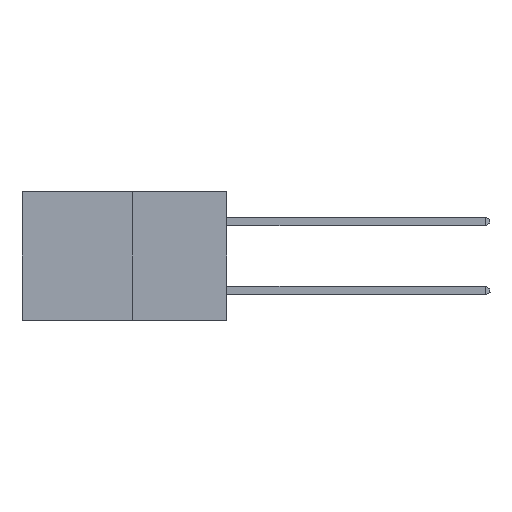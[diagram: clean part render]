
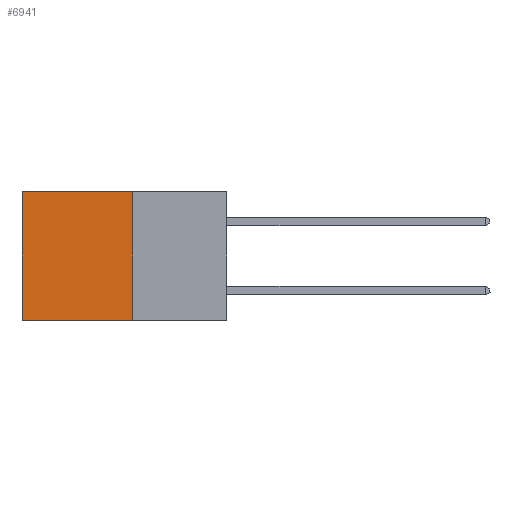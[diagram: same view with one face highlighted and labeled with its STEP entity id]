
A CAD part, left-side view. The second image highlights one B-rep face of the part: STEP entity #6941.
In plain terms, the highlighted planar face has unit normal (-1, 0, 0).
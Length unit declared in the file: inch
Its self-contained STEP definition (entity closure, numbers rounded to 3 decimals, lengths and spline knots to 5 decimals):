
#13 = CARTESIAN_POINT ( 'NONE',  ( 0.277, 0.27, 0. ) ) ;
#68 = LINE ( 'NONE', #5276, #3127 ) ;
#128 = ORIENTED_EDGE ( 'NONE', *, *, #6680, .T. ) ;
#270 = PLANE ( 'NONE',  #3419 ) ;
#528 = EDGE_CURVE ( 'NONE', #2380, #3860, #68, .T. ) ;
#669 = DIRECTION ( 'NONE',  ( 0., 1., 0. ) ) ;
#721 = DIRECTION ( 'NONE',  ( 0., 0., -1. ) ) ;
#1152 = ORIENTED_EDGE ( 'NONE', *, *, #3799, .F. ) ;
#1597 = DIRECTION ( 'NONE',  ( 0., 0., -1. ) ) ;
#1924 = DIRECTION ( 'NONE',  ( 0., 0., -1. ) ) ;
#2313 = CARTESIAN_POINT ( 'NONE',  ( 0.277, 0.27, -0.37 ) ) ;
#2352 = VECTOR ( 'NONE', #7194, 39.37008 ) ;
#2380 = VERTEX_POINT ( 'NONE', #2932 ) ;
#2598 = ORIENTED_EDGE ( 'NONE', *, *, #528, .T. ) ;
#2932 = CARTESIAN_POINT ( 'NONE',  ( 0.277, 0.59, 0. ) ) ;
#2978 = LINE ( 'NONE', #5140, #6423 ) ;
#3053 = ORIENTED_EDGE ( 'NONE', *, *, #7862, .F. ) ;
#3087 = VECTOR ( 'NONE', #669, 39.37008 ) ;
#3127 = VECTOR ( 'NONE', #721, 39.37008 ) ;
#3280 = CARTESIAN_POINT ( 'NONE',  ( 0.277, 0.59, -0.37 ) ) ;
#3419 = AXIS2_PLACEMENT_3D ( 'NONE', #4808, #5457, #1597 ) ;
#3799 = EDGE_CURVE ( 'NONE', #4544, #4170, #2978, .T. ) ;
#3860 = VERTEX_POINT ( 'NONE', #3280 ) ;
#4170 = VERTEX_POINT ( 'NONE', #2313 ) ;
#4544 = VERTEX_POINT ( 'NONE', #6530 ) ;
#4808 = CARTESIAN_POINT ( 'NONE',  ( 0.277, 0.27, -0.37 ) ) ;
#5140 = CARTESIAN_POINT ( 'NONE',  ( 0.277, 0.27, -0.37 ) ) ;
#5276 = CARTESIAN_POINT ( 'NONE',  ( 0.277, 0.59, -0.37 ) ) ;
#5457 = DIRECTION ( 'NONE',  ( 1., 0., 0. ) ) ;
#5590 = EDGE_LOOP ( 'NONE', ( #2598, #3053, #1152, #128 ) ) ;
#6423 = VECTOR ( 'NONE', #1924, 39.37008 ) ;
#6530 = CARTESIAN_POINT ( 'NONE',  ( 0.277, 0.27, 0. ) ) ;
#6541 = LINE ( 'NONE', #13, #3087 ) ;
#6576 = CARTESIAN_POINT ( 'NONE',  ( 0.277, 0.27, -0.37 ) ) ;
#6680 = EDGE_CURVE ( 'NONE', #4544, #2380, #6541, .T. ) ;
#6941 = ADVANCED_FACE ( 'NONE', ( #8102 ), #270, .F. ) ;
#7194 = DIRECTION ( 'NONE',  ( 0., 1., 0. ) ) ;
#7499 = LINE ( 'NONE', #6576, #2352 ) ;
#7862 = EDGE_CURVE ( 'NONE', #4170, #3860, #7499, .T. ) ;
#8102 = FACE_OUTER_BOUND ( 'NONE', #5590, .T. ) ;
